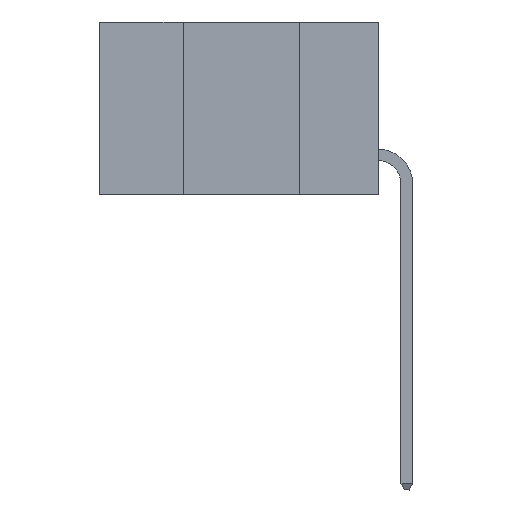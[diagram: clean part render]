
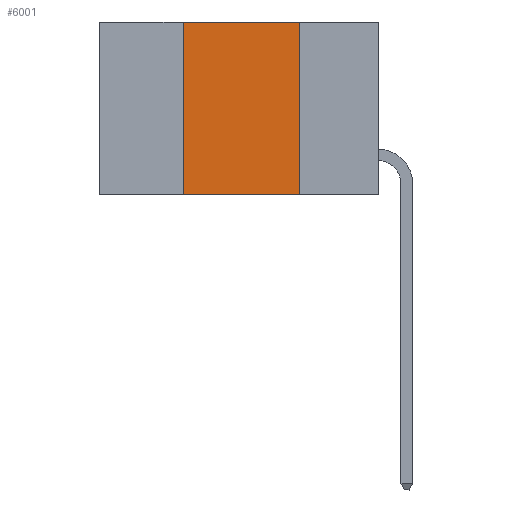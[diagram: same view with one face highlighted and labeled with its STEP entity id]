
A CAD part, left-side view. The second image highlights one B-rep face of the part: STEP entity #6001.
In plain terms, the highlighted planar face has unit normal (-1, 0, 0).
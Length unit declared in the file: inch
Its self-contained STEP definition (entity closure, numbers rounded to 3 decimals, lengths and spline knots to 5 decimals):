
#877 = ORIENTED_EDGE ( 'NONE', *, *, #3990, .T. ) ;
#1179 = LINE ( 'NONE', #13308, #1946 ) ;
#1523 = AXIS2_PLACEMENT_3D ( 'NONE', #3976, #4079, #15802 ) ;
#1946 = VECTOR ( 'NONE', #7270, 39.37008 ) ;
#2011 = ORIENTED_EDGE ( 'NONE', *, *, #6850, .F. ) ;
#2166 = VECTOR ( 'NONE', #9139, 39.37008 ) ;
#2257 = VERTEX_POINT ( 'NONE', #13077 ) ;
#3419 = EDGE_CURVE ( 'NONE', #13477, #13639, #12398, .T. ) ;
#3976 = CARTESIAN_POINT ( 'NONE',  ( 0., 0.6, 0. ) ) ;
#3990 = EDGE_CURVE ( 'NONE', #2257, #14373, #1179, .T. ) ;
#4079 = DIRECTION ( 'NONE',  ( 1., 0., 0. ) ) ;
#4178 = PLANE ( 'NONE',  #1523 ) ;
#6001 = ADVANCED_FACE ( 'NONE', ( #18906 ), #4178, .F. ) ;
#6850 = EDGE_CURVE ( 'NONE', #13639, #14373, #9371, .T. ) ;
#7130 = VECTOR ( 'NONE', #18279, 39.37008 ) ;
#7270 = DIRECTION ( 'NONE',  ( 0., -1., 0. ) ) ;
#7857 = CARTESIAN_POINT ( 'NONE',  ( 0., 0.17, -0.37 ) ) ;
#9139 = DIRECTION ( 'NONE',  ( 0., 0., 1. ) ) ;
#9225 = CARTESIAN_POINT ( 'NONE',  ( 0., 0.42, -0.37 ) ) ;
#9342 = VECTOR ( 'NONE', #12212, 39.37008 ) ;
#9371 = LINE ( 'NONE', #13854, #7130 ) ;
#11779 = EDGE_CURVE ( 'NONE', #2257, #13477, #16398, .T. ) ;
#12212 = DIRECTION ( 'NONE',  ( 0., -1., 0. ) ) ;
#12398 = LINE ( 'NONE', #15119, #9342 ) ;
#12992 = EDGE_LOOP ( 'NONE', ( #2011, #16368, #13530, #877 ) ) ;
#13077 = CARTESIAN_POINT ( 'NONE',  ( 0., 0.42, -0.37 ) ) ;
#13308 = CARTESIAN_POINT ( 'NONE',  ( 0., 0.6, -0.37 ) ) ;
#13477 = VERTEX_POINT ( 'NONE', #13559 ) ;
#13530 = ORIENTED_EDGE ( 'NONE', *, *, #11779, .F. ) ;
#13559 = CARTESIAN_POINT ( 'NONE',  ( 0., 0.42, 0. ) ) ;
#13639 = VERTEX_POINT ( 'NONE', #17192 ) ;
#13854 = CARTESIAN_POINT ( 'NONE',  ( 0., 0.17, -0.37 ) ) ;
#14373 = VERTEX_POINT ( 'NONE', #7857 ) ;
#15119 = CARTESIAN_POINT ( 'NONE',  ( 0., 0.6, 0. ) ) ;
#15802 = DIRECTION ( 'NONE',  ( 0., 0., -1. ) ) ;
#16368 = ORIENTED_EDGE ( 'NONE', *, *, #3419, .F. ) ;
#16398 = LINE ( 'NONE', #9225, #2166 ) ;
#17192 = CARTESIAN_POINT ( 'NONE',  ( 0., 0.17, 0. ) ) ;
#18279 = DIRECTION ( 'NONE',  ( 0., 0., -1. ) ) ;
#18906 = FACE_OUTER_BOUND ( 'NONE', #12992, .T. ) ;
